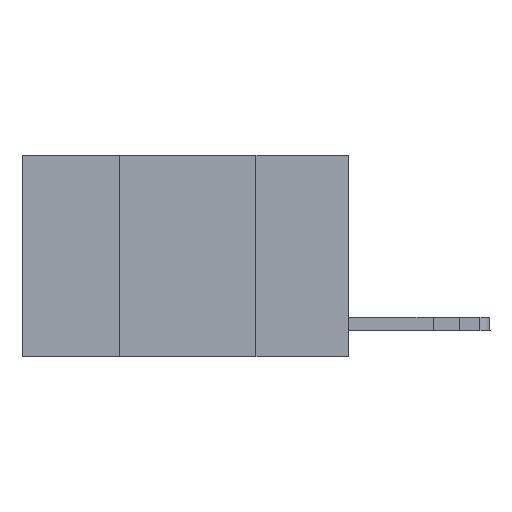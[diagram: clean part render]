
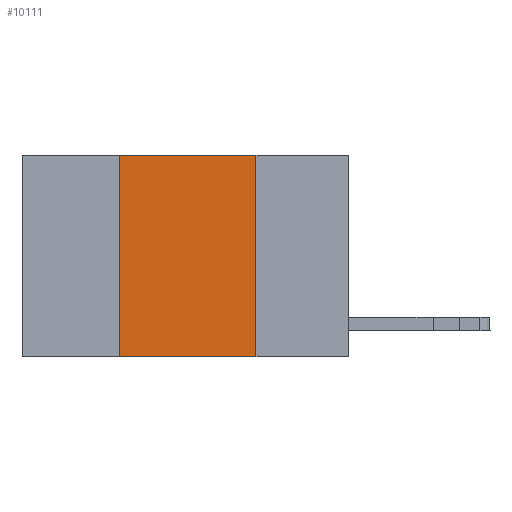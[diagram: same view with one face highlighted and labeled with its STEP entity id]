
A CAD part, left-side view. The second image highlights one B-rep face of the part: STEP entity #10111.
In plain terms, the highlighted planar face has unit normal (-1, 0, 0).
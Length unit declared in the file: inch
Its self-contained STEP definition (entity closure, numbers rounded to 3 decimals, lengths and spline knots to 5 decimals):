
#137 = DIRECTION ( 'NONE',  ( 0., -1., 0. ) ) ;
#599 = FACE_OUTER_BOUND ( 'NONE', #4358, .T. ) ;
#1299 = VERTEX_POINT ( 'NONE', #11211 ) ;
#1339 = VECTOR ( 'NONE', #137, 39.37008 ) ;
#2256 = VECTOR ( 'NONE', #13554, 39.37008 ) ;
#2493 = CARTESIAN_POINT ( 'NONE',  ( 0., 0.42, 0. ) ) ;
#2953 = VECTOR ( 'NONE', #5738, 39.37008 ) ;
#3575 = DIRECTION ( 'NONE',  ( 0., 0., 1. ) ) ;
#3711 = CARTESIAN_POINT ( 'NONE',  ( 0., 0.6, -0.37 ) ) ;
#3898 = CARTESIAN_POINT ( 'NONE',  ( 0., 0.6, 0. ) ) ;
#4358 = EDGE_LOOP ( 'NONE', ( #5814, #8686, #6139, #9049 ) ) ;
#4634 = CARTESIAN_POINT ( 'NONE',  ( 0., 0.17, 0. ) ) ;
#4939 = DIRECTION ( 'NONE',  ( 0., 0., -1. ) ) ;
#5080 = LINE ( 'NONE', #3711, #2256 ) ;
#5387 = AXIS2_PLACEMENT_3D ( 'NONE', #3898, #11541, #4939 ) ;
#5738 = DIRECTION ( 'NONE',  ( 0., 0., -1. ) ) ;
#5814 = ORIENTED_EDGE ( 'NONE', *, *, #8265, .F. ) ;
#5948 = VERTEX_POINT ( 'NONE', #7623 ) ;
#6139 = ORIENTED_EDGE ( 'NONE', *, *, #8248, .F. ) ;
#6419 = LINE ( 'NONE', #2493, #8989 ) ;
#7623 = CARTESIAN_POINT ( 'NONE',  ( 0., 0.42, 0. ) ) ;
#8248 = EDGE_CURVE ( 'NONE', #1299, #5948, #6419, .T. ) ;
#8265 = EDGE_CURVE ( 'NONE', #9070, #11214, #11990, .T. ) ;
#8329 = EDGE_CURVE ( 'NONE', #1299, #11214, #5080, .T. ) ;
#8686 = ORIENTED_EDGE ( 'NONE', *, *, #9286, .F. ) ;
#8989 = VECTOR ( 'NONE', #3575, 39.37008 ) ;
#9049 = ORIENTED_EDGE ( 'NONE', *, *, #8329, .T. ) ;
#9070 = VERTEX_POINT ( 'NONE', #12844 ) ;
#9267 = PLANE ( 'NONE',  #5387 ) ;
#9286 = EDGE_CURVE ( 'NONE', #5948, #9070, #10014, .T. ) ;
#10014 = LINE ( 'NONE', #13246, #1339 ) ;
#10111 = ADVANCED_FACE ( 'NONE', ( #599 ), #9267, .F. ) ;
#11177 = CARTESIAN_POINT ( 'NONE',  ( 0., 0.17, -0.37 ) ) ;
#11211 = CARTESIAN_POINT ( 'NONE',  ( 0., 0.42, -0.37 ) ) ;
#11214 = VERTEX_POINT ( 'NONE', #11177 ) ;
#11541 = DIRECTION ( 'NONE',  ( 1., 0., 0. ) ) ;
#11990 = LINE ( 'NONE', #4634, #2953 ) ;
#12844 = CARTESIAN_POINT ( 'NONE',  ( 0., 0.17, 0. ) ) ;
#13246 = CARTESIAN_POINT ( 'NONE',  ( 0., 0.6, 0. ) ) ;
#13554 = DIRECTION ( 'NONE',  ( 0., -1., 0. ) ) ;
